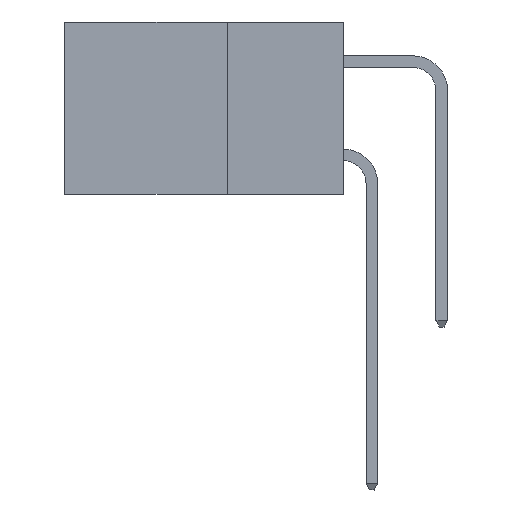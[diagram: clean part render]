
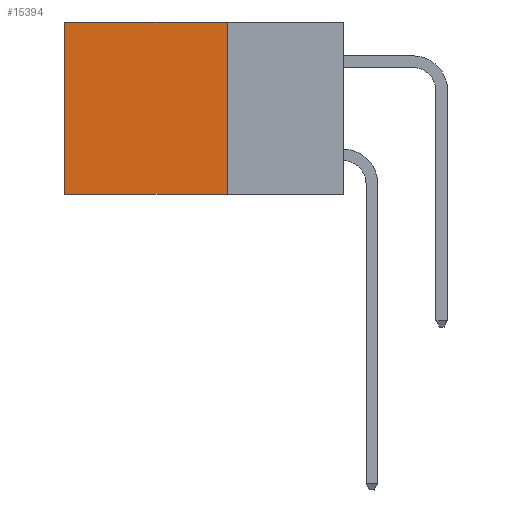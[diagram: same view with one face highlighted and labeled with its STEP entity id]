
A CAD part, left-side view. The second image highlights one B-rep face of the part: STEP entity #15394.
In plain terms, the highlighted planar face has unit normal (-1, 0, 0).
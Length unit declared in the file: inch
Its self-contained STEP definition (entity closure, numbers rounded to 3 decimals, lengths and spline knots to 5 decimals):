
#43 = LINE ( 'NONE', #10897, #6226 ) ;
#348 = EDGE_CURVE ( 'NONE', #2990, #1945, #14016, .T. ) ;
#516 = VERTEX_POINT ( 'NONE', #3426 ) ;
#1945 = VERTEX_POINT ( 'NONE', #14942 ) ;
#2567 = ORIENTED_EDGE ( 'NONE', *, *, #15344, .F. ) ;
#2990 = VERTEX_POINT ( 'NONE', #7739 ) ;
#3224 = VECTOR ( 'NONE', #11627, 39.37008 ) ;
#3276 = VECTOR ( 'NONE', #12408, 39.37008 ) ;
#3387 = EDGE_CURVE ( 'NONE', #2990, #10601, #6232, .T. ) ;
#3426 = CARTESIAN_POINT ( 'NONE',  ( 0.2615, 0.6, -0.37 ) ) ;
#4114 = DIRECTION ( 'NONE',  ( 0., 1., 0. ) ) ;
#4259 = CARTESIAN_POINT ( 'NONE',  ( 0.2615, 0.25, -0.37 ) ) ;
#6226 = VECTOR ( 'NONE', #4114, 39.37008 ) ;
#6232 = LINE ( 'NONE', #7759, #14661 ) ;
#6446 = CARTESIAN_POINT ( 'NONE',  ( 0.2615, 0.6, -0.37 ) ) ;
#7042 = ORIENTED_EDGE ( 'NONE', *, *, #3387, .F. ) ;
#7699 = LINE ( 'NONE', #6446, #3224 ) ;
#7739 = CARTESIAN_POINT ( 'NONE',  ( 0.2615, 0.25, 0. ) ) ;
#7759 = CARTESIAN_POINT ( 'NONE',  ( 0.2615, 0.25, -0.37 ) ) ;
#8450 = DIRECTION ( 'NONE',  ( 0., 0., -1. ) ) ;
#8547 = DIRECTION ( 'NONE',  ( 1., 0., 0. ) ) ;
#9662 = AXIS2_PLACEMENT_3D ( 'NONE', #15134, #8547, #8450 ) ;
#9971 = FACE_OUTER_BOUND ( 'NONE', #13763, .T. ) ;
#10359 = DIRECTION ( 'NONE',  ( 0., 0., -1. ) ) ;
#10601 = VERTEX_POINT ( 'NONE', #4259 ) ;
#10837 = ORIENTED_EDGE ( 'NONE', *, *, #11722, .T. ) ;
#10897 = CARTESIAN_POINT ( 'NONE',  ( 0.2615, 0.25, -0.37 ) ) ;
#11627 = DIRECTION ( 'NONE',  ( 0., 0., -1. ) ) ;
#11722 = EDGE_CURVE ( 'NONE', #1945, #516, #7699, .T. ) ;
#12408 = DIRECTION ( 'NONE',  ( 0., 1., 0. ) ) ;
#12489 = CARTESIAN_POINT ( 'NONE',  ( 0.2615, 0.25, 0. ) ) ;
#13223 = ORIENTED_EDGE ( 'NONE', *, *, #348, .T. ) ;
#13763 = EDGE_LOOP ( 'NONE', ( #10837, #2567, #7042, #13223 ) ) ;
#14016 = LINE ( 'NONE', #12489, #3276 ) ;
#14661 = VECTOR ( 'NONE', #10359, 39.37008 ) ;
#14942 = CARTESIAN_POINT ( 'NONE',  ( 0.2615, 0.6, 0. ) ) ;
#15134 = CARTESIAN_POINT ( 'NONE',  ( 0.2615, 0.25, -0.37 ) ) ;
#15344 = EDGE_CURVE ( 'NONE', #10601, #516, #43, .T. ) ;
#15381 = PLANE ( 'NONE',  #9662 ) ;
#15394 = ADVANCED_FACE ( 'NONE', ( #9971 ), #15381, .F. ) ;
